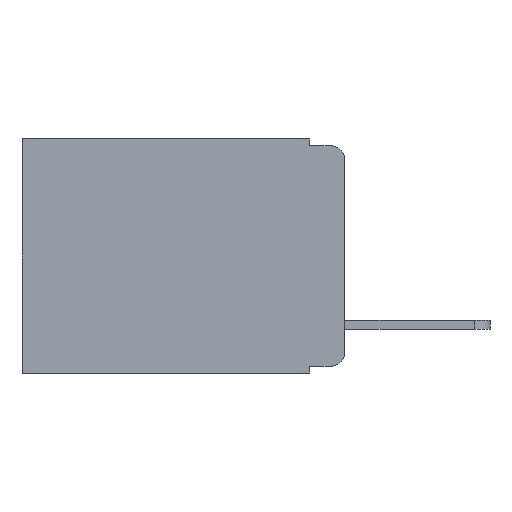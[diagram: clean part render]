
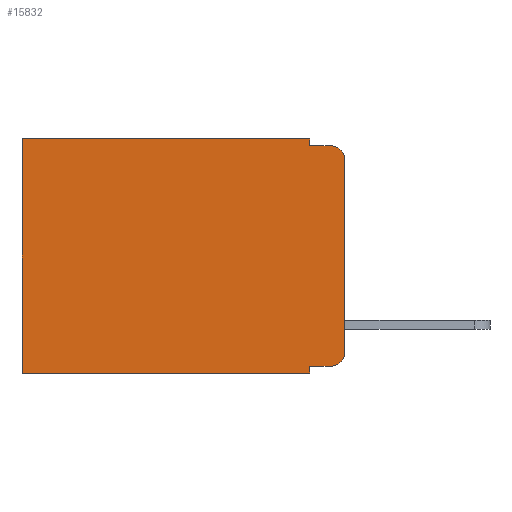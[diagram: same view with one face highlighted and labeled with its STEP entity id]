
A CAD part, left-side view. The second image highlights one B-rep face of the part: STEP entity #15832.
In plain terms, the highlighted planar face has unit normal (-1, 0, 0).
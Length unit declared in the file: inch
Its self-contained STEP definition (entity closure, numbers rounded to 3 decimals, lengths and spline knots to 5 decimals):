
#522 = LINE ( 'NONE', #2178, #5680 ) ;
#686 = LINE ( 'NONE', #1417, #14586 ) ;
#958 = LINE ( 'NONE', #5666, #9630 ) ;
#1073 = EDGE_CURVE ( 'NONE', #2976, #18370, #20038, .T. ) ;
#1310 = CARTESIAN_POINT ( 'NONE',  ( 0.298, 0., -0.343 ) ) ;
#1417 = CARTESIAN_POINT ( 'NONE',  ( 0.298, 0.051, -0.333 ) ) ;
#1669 = ORIENTED_EDGE ( 'NONE', *, *, #5038, .F. ) ;
#2140 = DIRECTION ( 'NONE',  ( 0., 0., -1. ) ) ;
#2178 = CARTESIAN_POINT ( 'NONE',  ( 0.298, 0.051, 0. ) ) ;
#2234 = VERTEX_POINT ( 'NONE', #14562 ) ;
#2301 = VERTEX_POINT ( 'NONE', #3579 ) ;
#2976 = VERTEX_POINT ( 'NONE', #12524 ) ;
#3579 = CARTESIAN_POINT ( 'NONE',  ( 0.298, 0.473, 0. ) ) ;
#3749 = ORIENTED_EDGE ( 'NONE', *, *, #10312, .T. ) ;
#4096 = VECTOR ( 'NONE', #14883, 39.37008 ) ;
#4149 = CARTESIAN_POINT ( 'NONE',  ( 0.298, 0.051, 0. ) ) ;
#4188 = PLANE ( 'NONE',  #5901 ) ;
#4219 = EDGE_CURVE ( 'NONE', #4584, #18529, #686, .T. ) ;
#4430 = EDGE_CURVE ( 'NONE', #4584, #15424, #6396, .T. ) ;
#4584 = VERTEX_POINT ( 'NONE', #6037 ) ;
#5038 = EDGE_CURVE ( 'NONE', #2234, #13463, #5250, .T. ) ;
#5120 = CARTESIAN_POINT ( 'NONE',  ( 0.298, 0.02, -0.313 ) ) ;
#5250 = LINE ( 'NONE', #18467, #4096 ) ;
#5666 = CARTESIAN_POINT ( 'NONE',  ( 0.298, 0.473, 0. ) ) ;
#5680 = VECTOR ( 'NONE', #11089, 39.37008 ) ;
#5729 = VECTOR ( 'NONE', #14651, 39.37008 ) ;
#5889 = DIRECTION ( 'NONE',  ( -1., 0., 0. ) ) ;
#5901 = AXIS2_PLACEMENT_3D ( 'NONE', #20923, #18793, #18940 ) ;
#6037 = CARTESIAN_POINT ( 'NONE',  ( 0.298, 0.051, -0.333 ) ) ;
#6396 = LINE ( 'NONE', #18078, #14285 ) ;
#6861 = AXIS2_PLACEMENT_3D ( 'NONE', #5120, #9610, #12649 ) ;
#7287 = EDGE_CURVE ( 'NONE', #22464, #2234, #522, .T. ) ;
#7692 = DIRECTION ( 'NONE',  ( 0., 0., -1. ) ) ;
#9610 = DIRECTION ( 'NONE',  ( -1., 0., 0. ) ) ;
#9630 = VECTOR ( 'NONE', #7692, 39.37008 ) ;
#9771 = ORIENTED_EDGE ( 'NONE', *, *, #4219, .T. ) ;
#10088 = EDGE_LOOP ( 'NONE', ( #21279, #3749, #1669, #13215, #14494, #19722, #22221, #20705, #9771, #22990 ) ) ;
#10312 = EDGE_CURVE ( 'NONE', #2976, #13463, #12351, .T. ) ;
#10842 = CARTESIAN_POINT ( 'NONE',  ( 0.298, 0.02, -0.333 ) ) ;
#11089 = DIRECTION ( 'NONE',  ( 0., 0., -1. ) ) ;
#12351 = CIRCLE ( 'NONE', #23363, 0.02 ) ;
#12524 = CARTESIAN_POINT ( 'NONE',  ( 0.298, 0., -0.03 ) ) ;
#12649 = DIRECTION ( 'NONE',  ( 0., 0., -1. ) ) ;
#13024 = VERTEX_POINT ( 'NONE', #18787 ) ;
#13193 = CARTESIAN_POINT ( 'NONE',  ( 0.298, 0.051, -0.343 ) ) ;
#13215 = ORIENTED_EDGE ( 'NONE', *, *, #7287, .F. ) ;
#13463 = VERTEX_POINT ( 'NONE', #22749 ) ;
#13925 = VECTOR ( 'NONE', #23265, 39.37008 ) ;
#14114 = CARTESIAN_POINT ( 'NONE',  ( 0.298, 0., -0.313 ) ) ;
#14285 = VECTOR ( 'NONE', #17933, 39.37008 ) ;
#14494 = ORIENTED_EDGE ( 'NONE', *, *, #15782, .T. ) ;
#14562 = CARTESIAN_POINT ( 'NONE',  ( 0.298, 0.051, -0.01 ) ) ;
#14586 = VECTOR ( 'NONE', #16217, 39.37008 ) ;
#14598 = VECTOR ( 'NONE', #2140, 39.37008 ) ;
#14619 = EDGE_CURVE ( 'NONE', #15424, #13024, #17969, .T. ) ;
#14651 = DIRECTION ( 'NONE',  ( 0., 1., 0. ) ) ;
#14883 = DIRECTION ( 'NONE',  ( 0., -1., 0. ) ) ;
#15314 = LINE ( 'NONE', #23687, #5729 ) ;
#15403 = DIRECTION ( 'NONE',  ( 0., 0., -1. ) ) ;
#15424 = VERTEX_POINT ( 'NONE', #13193 ) ;
#15782 = EDGE_CURVE ( 'NONE', #22464, #2301, #15314, .T. ) ;
#15832 = ADVANCED_FACE ( 'NONE', ( #19919 ), #4188, .F. ) ;
#16217 = DIRECTION ( 'NONE',  ( 0., -1., 0. ) ) ;
#16745 = EDGE_CURVE ( 'NONE', #18529, #18370, #17996, .T. ) ;
#16938 = EDGE_CURVE ( 'NONE', #2301, #13024, #958, .T. ) ;
#17933 = DIRECTION ( 'NONE',  ( 0., 0., -1. ) ) ;
#17969 = LINE ( 'NONE', #1310, #13925 ) ;
#17996 = CIRCLE ( 'NONE', #6861, 0.02 ) ;
#18078 = CARTESIAN_POINT ( 'NONE',  ( 0.298, 0.051, 0. ) ) ;
#18370 = VERTEX_POINT ( 'NONE', #14114 ) ;
#18467 = CARTESIAN_POINT ( 'NONE',  ( 0.298, 0.051, -0.01 ) ) ;
#18529 = VERTEX_POINT ( 'NONE', #10842 ) ;
#18787 = CARTESIAN_POINT ( 'NONE',  ( 0.298, 0.473, -0.343 ) ) ;
#18793 = DIRECTION ( 'NONE',  ( 1., 0., 0. ) ) ;
#18940 = DIRECTION ( 'NONE',  ( 0., 0., -1. ) ) ;
#19162 = CARTESIAN_POINT ( 'NONE',  ( 0.298, 0.02, -0.03 ) ) ;
#19722 = ORIENTED_EDGE ( 'NONE', *, *, #16938, .T. ) ;
#19919 = FACE_OUTER_BOUND ( 'NONE', #10088, .T. ) ;
#20038 = LINE ( 'NONE', #20560, #14598 ) ;
#20560 = CARTESIAN_POINT ( 'NONE',  ( 0.298, 0., 0. ) ) ;
#20705 = ORIENTED_EDGE ( 'NONE', *, *, #4430, .F. ) ;
#20923 = CARTESIAN_POINT ( 'NONE',  ( 0.298, 0., 0. ) ) ;
#21279 = ORIENTED_EDGE ( 'NONE', *, *, #1073, .F. ) ;
#22221 = ORIENTED_EDGE ( 'NONE', *, *, #14619, .F. ) ;
#22464 = VERTEX_POINT ( 'NONE', #4149 ) ;
#22749 = CARTESIAN_POINT ( 'NONE',  ( 0.298, 0.02, -0.01 ) ) ;
#22990 = ORIENTED_EDGE ( 'NONE', *, *, #16745, .T. ) ;
#23265 = DIRECTION ( 'NONE',  ( 0., 1., 0. ) ) ;
#23363 = AXIS2_PLACEMENT_3D ( 'NONE', #19162, #5889, #15403 ) ;
#23687 = CARTESIAN_POINT ( 'NONE',  ( 0.298, 0., 0. ) ) ;
